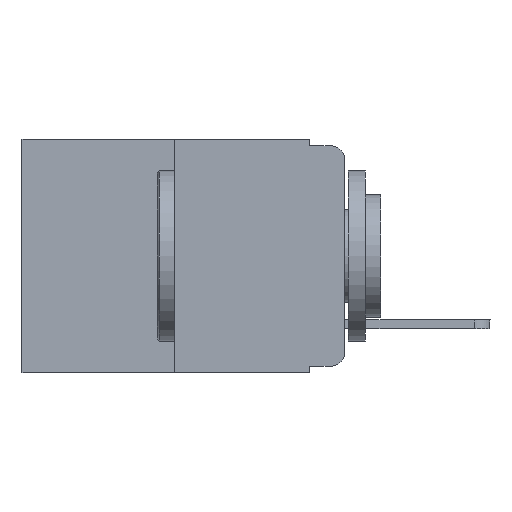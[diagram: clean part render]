
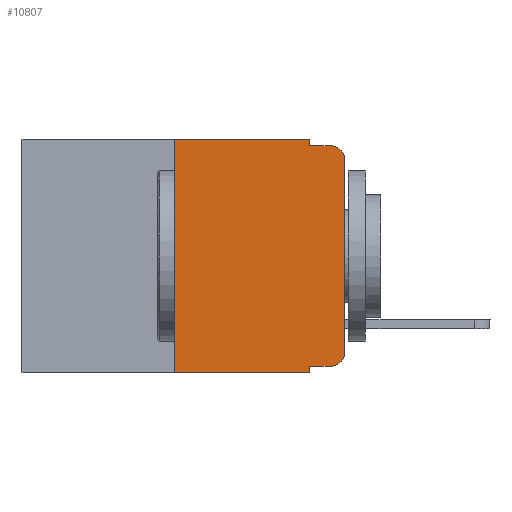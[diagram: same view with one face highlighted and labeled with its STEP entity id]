
A CAD part, left-side view. The second image highlights one B-rep face of the part: STEP entity #10807.
In plain terms, the highlighted planar face has unit normal (-1, 0, 0).
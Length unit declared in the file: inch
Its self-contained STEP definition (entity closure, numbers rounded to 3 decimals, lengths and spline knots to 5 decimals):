
#18 = VERTEX_POINT ( 'NONE', #4590 ) ;
#45 = DIRECTION ( 'NONE',  ( 0., 0., -1. ) ) ;
#445 = VERTEX_POINT ( 'NONE', #7018 ) ;
#586 = ORIENTED_EDGE ( 'NONE', *, *, #2158, .F. ) ;
#628 = CARTESIAN_POINT ( 'NONE',  ( 0., 0.051, -0.343 ) ) ;
#1072 = VERTEX_POINT ( 'NONE', #3468 ) ;
#1146 = CARTESIAN_POINT ( 'NONE',  ( 0., 0.473, -0.343 ) ) ;
#1251 = LINE ( 'NONE', #7211, #9823 ) ;
#1487 = CIRCLE ( 'NONE', #4779, 0.02 ) ;
#1885 = VECTOR ( 'NONE', #2532, 39.37008 ) ;
#1980 = EDGE_CURVE ( 'NONE', #6953, #10727, #10450, .T. ) ;
#1994 = DIRECTION ( 'NONE',  ( 0., 0., -1. ) ) ;
#2100 = EDGE_CURVE ( 'NONE', #445, #18, #2812, .T. ) ;
#2129 = VERTEX_POINT ( 'NONE', #628 ) ;
#2131 = DIRECTION ( 'NONE',  ( 0., -1., 0. ) ) ;
#2158 = EDGE_CURVE ( 'NONE', #2430, #2129, #4515, .T. ) ;
#2342 = CARTESIAN_POINT ( 'NONE',  ( 0., 0.02, -0.01 ) ) ;
#2430 = VERTEX_POINT ( 'NONE', #9873 ) ;
#2532 = DIRECTION ( 'NONE',  ( 0., 0., -1. ) ) ;
#2597 = VECTOR ( 'NONE', #3962, 39.37008 ) ;
#2618 = CARTESIAN_POINT ( 'NONE',  ( 0., 0.25, 0. ) ) ;
#2671 = DIRECTION ( 'NONE',  ( 0., 0., -1. ) ) ;
#2710 = EDGE_CURVE ( 'NONE', #2430, #1072, #6187, .T. ) ;
#2812 = LINE ( 'NONE', #11398, #9520 ) ;
#2891 = LINE ( 'NONE', #11879, #4909 ) ;
#3468 = CARTESIAN_POINT ( 'NONE',  ( 0., 0.02, -0.333 ) ) ;
#3693 = CARTESIAN_POINT ( 'NONE',  ( 0., 0.02, -0.03 ) ) ;
#3733 = DIRECTION ( 'NONE',  ( 0., 0., 1. ) ) ;
#3801 = CARTESIAN_POINT ( 'NONE',  ( 0., 0.051, 0. ) ) ;
#3962 = DIRECTION ( 'NONE',  ( 0., -1., 0. ) ) ;
#4420 = CARTESIAN_POINT ( 'NONE',  ( 0., 0.25, 0. ) ) ;
#4449 = LINE ( 'NONE', #1146, #5825 ) ;
#4515 = LINE ( 'NONE', #9553, #1885 ) ;
#4590 = CARTESIAN_POINT ( 'NONE',  ( 0., 0., -0.03 ) ) ;
#4669 = ORIENTED_EDGE ( 'NONE', *, *, #9806, .T. ) ;
#4779 = AXIS2_PLACEMENT_3D ( 'NONE', #5038, #5859, #1994 ) ;
#4909 = VECTOR ( 'NONE', #45, 39.37008 ) ;
#5038 = CARTESIAN_POINT ( 'NONE',  ( 0., 0.02, -0.313 ) ) ;
#5116 = AXIS2_PLACEMENT_3D ( 'NONE', #9719, #5719, #7418 ) ;
#5216 = LINE ( 'NONE', #10006, #2597 ) ;
#5719 = DIRECTION ( 'NONE',  ( 1., 0., 0. ) ) ;
#5825 = VECTOR ( 'NONE', #9117, 39.37008 ) ;
#5839 = EDGE_CURVE ( 'NONE', #10727, #6309, #1251, .T. ) ;
#5859 = DIRECTION ( 'NONE',  ( -1., 0., 0. ) ) ;
#5960 = EDGE_LOOP ( 'NONE', ( #10733, #12221, #10717, #7718, #11083, #10683, #9154, #586, #9819, #4669 ) ) ;
#6187 = LINE ( 'NONE', #11850, #11650 ) ;
#6309 = VERTEX_POINT ( 'NONE', #3801 ) ;
#6605 = DIRECTION ( 'NONE',  ( -1., 0., 0. ) ) ;
#6953 = VERTEX_POINT ( 'NONE', #12566 ) ;
#7018 = CARTESIAN_POINT ( 'NONE',  ( 0., 0., -0.313 ) ) ;
#7211 = CARTESIAN_POINT ( 'NONE',  ( 0., 0.473, 0. ) ) ;
#7418 = DIRECTION ( 'NONE',  ( 0., 0., -1. ) ) ;
#7434 = DIRECTION ( 'NONE',  ( 0., 0., 1. ) ) ;
#7503 = VERTEX_POINT ( 'NONE', #9621 ) ;
#7718 = ORIENTED_EDGE ( 'NONE', *, *, #9093, .F. ) ;
#8499 = CIRCLE ( 'NONE', #9725, 0.02 ) ;
#8677 = FACE_OUTER_BOUND ( 'NONE', #5960, .T. ) ;
#9093 = EDGE_CURVE ( 'NONE', #6309, #7503, #2891, .T. ) ;
#9117 = DIRECTION ( 'NONE',  ( 0., -1., 0. ) ) ;
#9154 = ORIENTED_EDGE ( 'NONE', *, *, #9333, .T. ) ;
#9204 = VECTOR ( 'NONE', #3733, 39.37008 ) ;
#9333 = EDGE_CURVE ( 'NONE', #6953, #2129, #4449, .T. ) ;
#9520 = VECTOR ( 'NONE', #7434, 39.37008 ) ;
#9553 = CARTESIAN_POINT ( 'NONE',  ( 0., 0.051, 0. ) ) ;
#9588 = EDGE_CURVE ( 'NONE', #18, #12400, #8499, .T. ) ;
#9621 = CARTESIAN_POINT ( 'NONE',  ( 0., 0.051, -0.01 ) ) ;
#9719 = CARTESIAN_POINT ( 'NONE',  ( 0., 0.473, 0. ) ) ;
#9725 = AXIS2_PLACEMENT_3D ( 'NONE', #3693, #6605, #2671 ) ;
#9806 = EDGE_CURVE ( 'NONE', #1072, #445, #1487, .T. ) ;
#9819 = ORIENTED_EDGE ( 'NONE', *, *, #2710, .T. ) ;
#9823 = VECTOR ( 'NONE', #2131, 39.37008 ) ;
#9873 = CARTESIAN_POINT ( 'NONE',  ( 0., 0.051, -0.333 ) ) ;
#10006 = CARTESIAN_POINT ( 'NONE',  ( 0., 0.051, -0.01 ) ) ;
#10450 = LINE ( 'NONE', #2618, #9204 ) ;
#10683 = ORIENTED_EDGE ( 'NONE', *, *, #1980, .F. ) ;
#10717 = ORIENTED_EDGE ( 'NONE', *, *, #10931, .F. ) ;
#10727 = VERTEX_POINT ( 'NONE', #4420 ) ;
#10733 = ORIENTED_EDGE ( 'NONE', *, *, #2100, .T. ) ;
#10807 = ADVANCED_FACE ( 'NONE', ( #8677 ), #11692, .F. ) ;
#10931 = EDGE_CURVE ( 'NONE', #7503, #12400, #5216, .T. ) ;
#11083 = ORIENTED_EDGE ( 'NONE', *, *, #5839, .F. ) ;
#11398 = CARTESIAN_POINT ( 'NONE',  ( 0., 0., 0. ) ) ;
#11650 = VECTOR ( 'NONE', #12606, 39.37008 ) ;
#11692 = PLANE ( 'NONE',  #5116 ) ;
#11850 = CARTESIAN_POINT ( 'NONE',  ( 0., 0.051, -0.333 ) ) ;
#11879 = CARTESIAN_POINT ( 'NONE',  ( 0., 0.051, 0. ) ) ;
#12221 = ORIENTED_EDGE ( 'NONE', *, *, #9588, .T. ) ;
#12400 = VERTEX_POINT ( 'NONE', #2342 ) ;
#12566 = CARTESIAN_POINT ( 'NONE',  ( 0., 0.25, -0.343 ) ) ;
#12606 = DIRECTION ( 'NONE',  ( 0., -1., 0. ) ) ;
